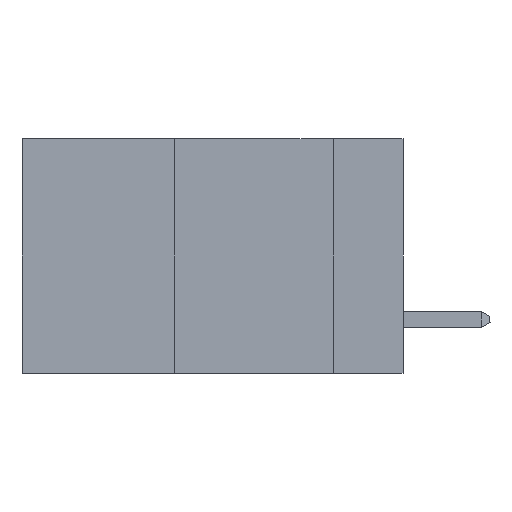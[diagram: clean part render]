
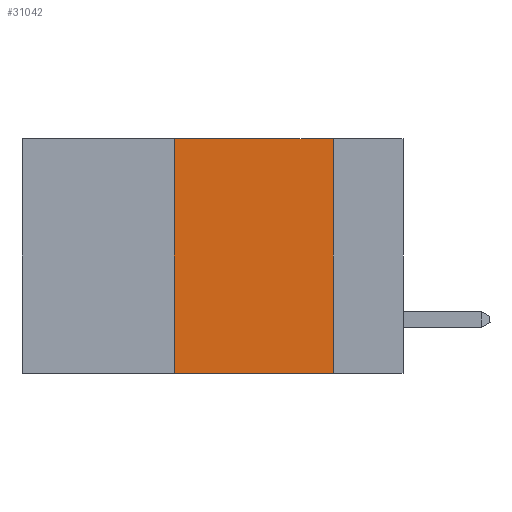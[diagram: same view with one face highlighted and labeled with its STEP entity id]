
A CAD part, left-side view. The second image highlights one B-rep face of the part: STEP entity #31042.
In plain terms, the highlighted planar face has unit normal (-1, 0, 0).
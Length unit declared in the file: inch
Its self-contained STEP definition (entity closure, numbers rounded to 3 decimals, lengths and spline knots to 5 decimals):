
#505 = CARTESIAN_POINT ( 'NONE',  ( 0., 0.6, 0. ) ) ;
#3072 = CARTESIAN_POINT ( 'NONE',  ( 0., 0.11, -0.37 ) ) ;
#3269 = EDGE_LOOP ( 'NONE', ( #19719, #22181, #33103, #8007 ) ) ;
#3984 = DIRECTION ( 'NONE',  ( 0., 0., -1. ) ) ;
#4198 = CARTESIAN_POINT ( 'NONE',  ( 0., 0.11, 0. ) ) ;
#5483 = LINE ( 'NONE', #23906, #6299 ) ;
#5509 = LINE ( 'NONE', #7787, #22645 ) ;
#6299 = VECTOR ( 'NONE', #13503, 39.37008 ) ;
#7570 = DIRECTION ( 'NONE',  ( 0., 0., -1. ) ) ;
#7787 = CARTESIAN_POINT ( 'NONE',  ( 0., 0.6, -0.37 ) ) ;
#8007 = ORIENTED_EDGE ( 'NONE', *, *, #28273, .T. ) ;
#8664 = CARTESIAN_POINT ( 'NONE',  ( 0., 0.36, 0. ) ) ;
#11688 = LINE ( 'NONE', #14141, #14950 ) ;
#12228 = VERTEX_POINT ( 'NONE', #8664 ) ;
#12445 = CARTESIAN_POINT ( 'NONE',  ( 0., 0.6, 0. ) ) ;
#12778 = DIRECTION ( 'NONE',  ( 0., -1., 0. ) ) ;
#13247 = VERTEX_POINT ( 'NONE', #27255 ) ;
#13503 = DIRECTION ( 'NONE',  ( 0., 0., 1. ) ) ;
#14141 = CARTESIAN_POINT ( 'NONE',  ( 0., 0.11, 0. ) ) ;
#14328 = VERTEX_POINT ( 'NONE', #3072 ) ;
#14950 = VECTOR ( 'NONE', #3984, 39.37008 ) ;
#16951 = VECTOR ( 'NONE', #24288, 39.37008 ) ;
#17674 = PLANE ( 'NONE',  #28524 ) ;
#18125 = LINE ( 'NONE', #505, #16951 ) ;
#19624 = FACE_OUTER_BOUND ( 'NONE', #3269, .T. ) ;
#19719 = ORIENTED_EDGE ( 'NONE', *, *, #27127, .F. ) ;
#20434 = DIRECTION ( 'NONE',  ( 1., 0., 0. ) ) ;
#22181 = ORIENTED_EDGE ( 'NONE', *, *, #22305, .F. ) ;
#22305 = EDGE_CURVE ( 'NONE', #12228, #33000, #18125, .T. ) ;
#22645 = VECTOR ( 'NONE', #12778, 39.37008 ) ;
#23906 = CARTESIAN_POINT ( 'NONE',  ( 0., 0.36, 0. ) ) ;
#24288 = DIRECTION ( 'NONE',  ( 0., -1., 0. ) ) ;
#27127 = EDGE_CURVE ( 'NONE', #33000, #14328, #11688, .T. ) ;
#27255 = CARTESIAN_POINT ( 'NONE',  ( 0., 0.36, -0.37 ) ) ;
#28273 = EDGE_CURVE ( 'NONE', #13247, #14328, #5509, .T. ) ;
#28524 = AXIS2_PLACEMENT_3D ( 'NONE', #12445, #20434, #7570 ) ;
#28586 = EDGE_CURVE ( 'NONE', #13247, #12228, #5483, .T. ) ;
#31042 = ADVANCED_FACE ( 'NONE', ( #19624 ), #17674, .F. ) ;
#33000 = VERTEX_POINT ( 'NONE', #4198 ) ;
#33103 = ORIENTED_EDGE ( 'NONE', *, *, #28586, .F. ) ;
